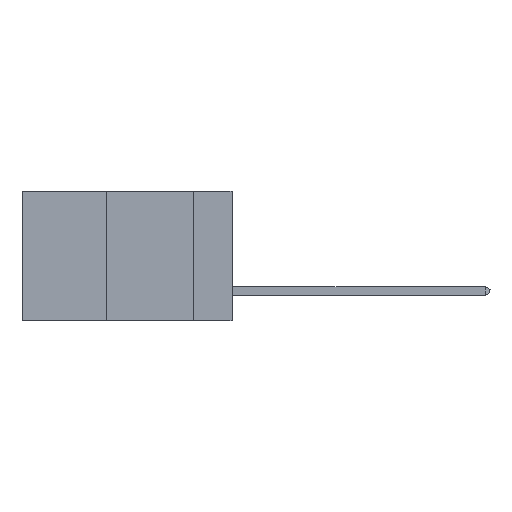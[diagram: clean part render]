
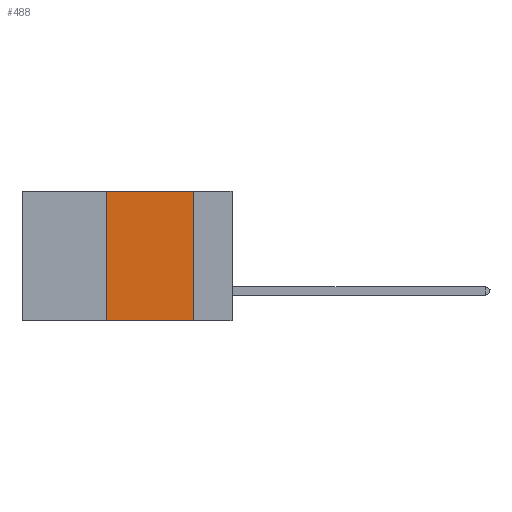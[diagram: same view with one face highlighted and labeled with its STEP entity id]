
A CAD part, left-side view. The second image highlights one B-rep face of the part: STEP entity #488.
In plain terms, the highlighted planar face has unit normal (-1, 0, 0).
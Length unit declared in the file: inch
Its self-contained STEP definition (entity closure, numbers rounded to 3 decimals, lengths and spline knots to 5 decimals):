
#254 = ORIENTED_EDGE ( 'NONE', *, *, #1604, .F. ) ;
#488 = ADVANCED_FACE ( 'NONE', ( #8388 ), #2938, .F. ) ;
#826 = LINE ( 'NONE', #1776, #1133 ) ;
#977 = CARTESIAN_POINT ( 'NONE',  ( 0., 0.6, 0. ) ) ;
#1113 = VECTOR ( 'NONE', #8585, 39.37008 ) ;
#1133 = VECTOR ( 'NONE', #8801, 39.37008 ) ;
#1328 = DIRECTION ( 'NONE',  ( 0., 0., -1. ) ) ;
#1544 = CARTESIAN_POINT ( 'NONE',  ( 0., 0.11, 0. ) ) ;
#1604 = EDGE_CURVE ( 'NONE', #9929, #8883, #826, .T. ) ;
#1605 = VERTEX_POINT ( 'NONE', #4791 ) ;
#1776 = CARTESIAN_POINT ( 'NONE',  ( 0., 0.36, 0. ) ) ;
#2132 = AXIS2_PLACEMENT_3D ( 'NONE', #977, #3023, #1328 ) ;
#2693 = CARTESIAN_POINT ( 'NONE',  ( 0., 0.36, -0.37 ) ) ;
#2938 = PLANE ( 'NONE',  #2132 ) ;
#3023 = DIRECTION ( 'NONE',  ( 1., 0., 0. ) ) ;
#3734 = VERTEX_POINT ( 'NONE', #8856 ) ;
#4791 = CARTESIAN_POINT ( 'NONE',  ( 0., 0.11, -0.37 ) ) ;
#4896 = VECTOR ( 'NONE', #11590, 39.37008 ) ;
#5325 = ORIENTED_EDGE ( 'NONE', *, *, #6131, .T. ) ;
#5727 = EDGE_LOOP ( 'NONE', ( #6101, #11618, #254, #5325 ) ) ;
#6101 = ORIENTED_EDGE ( 'NONE', *, *, #11368, .F. ) ;
#6131 = EDGE_CURVE ( 'NONE', #9929, #1605, #12829, .T. ) ;
#8388 = FACE_OUTER_BOUND ( 'NONE', #5727, .T. ) ;
#8474 = CARTESIAN_POINT ( 'NONE',  ( 0., 0.6, -0.37 ) ) ;
#8585 = DIRECTION ( 'NONE',  ( 0., 0., -1. ) ) ;
#8801 = DIRECTION ( 'NONE',  ( 0., 0., 1. ) ) ;
#8856 = CARTESIAN_POINT ( 'NONE',  ( 0., 0.11, 0. ) ) ;
#8875 = VECTOR ( 'NONE', #9618, 39.37008 ) ;
#8883 = VERTEX_POINT ( 'NONE', #12190 ) ;
#9136 = LINE ( 'NONE', #1544, #1113 ) ;
#9618 = DIRECTION ( 'NONE',  ( 0., -1., 0. ) ) ;
#9929 = VERTEX_POINT ( 'NONE', #2693 ) ;
#10566 = LINE ( 'NONE', #12461, #4896 ) ;
#10689 = EDGE_CURVE ( 'NONE', #8883, #3734, #10566, .T. ) ;
#11368 = EDGE_CURVE ( 'NONE', #3734, #1605, #9136, .T. ) ;
#11590 = DIRECTION ( 'NONE',  ( 0., -1., 0. ) ) ;
#11618 = ORIENTED_EDGE ( 'NONE', *, *, #10689, .F. ) ;
#12190 = CARTESIAN_POINT ( 'NONE',  ( 0., 0.36, 0. ) ) ;
#12461 = CARTESIAN_POINT ( 'NONE',  ( 0., 0.6, 0. ) ) ;
#12829 = LINE ( 'NONE', #8474, #8875 ) ;
